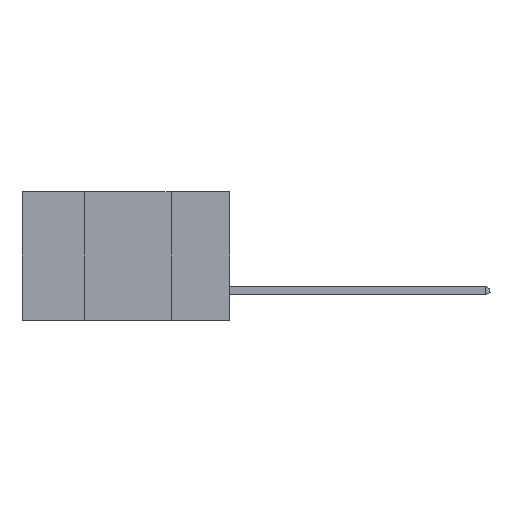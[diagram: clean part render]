
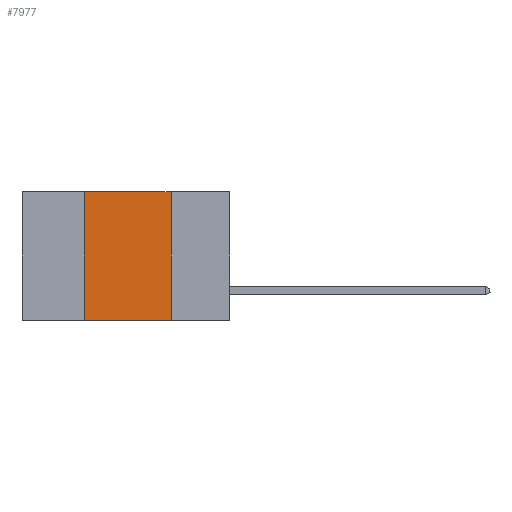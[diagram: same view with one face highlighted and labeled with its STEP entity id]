
A CAD part, left-side view. The second image highlights one B-rep face of the part: STEP entity #7977.
In plain terms, the highlighted planar face has unit normal (-1, 0, 0).
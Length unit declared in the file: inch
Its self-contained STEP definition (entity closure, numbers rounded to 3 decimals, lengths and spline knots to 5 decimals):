
#239 = VERTEX_POINT ( 'NONE', #2856 ) ;
#343 = EDGE_CURVE ( 'NONE', #239, #14109, #8706, .T. ) ;
#652 = VERTEX_POINT ( 'NONE', #15212 ) ;
#1117 = LINE ( 'NONE', #10203, #15800 ) ;
#1654 = VECTOR ( 'NONE', #10891, 39.37008 ) ;
#2674 = DIRECTION ( 'NONE',  ( 0., 0., -1. ) ) ;
#2856 = CARTESIAN_POINT ( 'NONE',  ( 0., 0.42, 0. ) ) ;
#3702 = ORIENTED_EDGE ( 'NONE', *, *, #10461, .T. ) ;
#3915 = ORIENTED_EDGE ( 'NONE', *, *, #6969, .F. ) ;
#4906 = AXIS2_PLACEMENT_3D ( 'NONE', #9082, #7619, #2674 ) ;
#5778 = CARTESIAN_POINT ( 'NONE',  ( 0., 0.17, 0. ) ) ;
#5860 = CARTESIAN_POINT ( 'NONE',  ( 0., 0.6, -0.37 ) ) ;
#6131 = FACE_OUTER_BOUND ( 'NONE', #7118, .T. ) ;
#6328 = PLANE ( 'NONE',  #4906 ) ;
#6969 = EDGE_CURVE ( 'NONE', #14109, #652, #8260, .T. ) ;
#7118 = EDGE_LOOP ( 'NONE', ( #3915, #11951, #8737, #3702 ) ) ;
#7619 = DIRECTION ( 'NONE',  ( 1., 0., 0. ) ) ;
#7655 = EDGE_CURVE ( 'NONE', #8499, #239, #1117, .T. ) ;
#7977 = ADVANCED_FACE ( 'NONE', ( #6131 ), #6328, .F. ) ;
#8260 = LINE ( 'NONE', #14717, #9081 ) ;
#8499 = VERTEX_POINT ( 'NONE', #16238 ) ;
#8671 = DIRECTION ( 'NONE',  ( 0., -1., 0. ) ) ;
#8706 = LINE ( 'NONE', #15983, #1654 ) ;
#8737 = ORIENTED_EDGE ( 'NONE', *, *, #7655, .F. ) ;
#9073 = LINE ( 'NONE', #5860, #13459 ) ;
#9081 = VECTOR ( 'NONE', #12280, 39.37008 ) ;
#9082 = CARTESIAN_POINT ( 'NONE',  ( 0., 0.6, 0. ) ) ;
#10203 = CARTESIAN_POINT ( 'NONE',  ( 0., 0.42, 0. ) ) ;
#10461 = EDGE_CURVE ( 'NONE', #8499, #652, #9073, .T. ) ;
#10891 = DIRECTION ( 'NONE',  ( 0., -1., 0. ) ) ;
#11951 = ORIENTED_EDGE ( 'NONE', *, *, #343, .F. ) ;
#12280 = DIRECTION ( 'NONE',  ( 0., 0., -1. ) ) ;
#13459 = VECTOR ( 'NONE', #8671, 39.37008 ) ;
#14109 = VERTEX_POINT ( 'NONE', #5778 ) ;
#14717 = CARTESIAN_POINT ( 'NONE',  ( 0., 0.17, 0. ) ) ;
#15212 = CARTESIAN_POINT ( 'NONE',  ( 0., 0.17, -0.37 ) ) ;
#15800 = VECTOR ( 'NONE', #15895, 39.37008 ) ;
#15895 = DIRECTION ( 'NONE',  ( 0., 0., 1. ) ) ;
#15983 = CARTESIAN_POINT ( 'NONE',  ( 0., 0.6, 0. ) ) ;
#16238 = CARTESIAN_POINT ( 'NONE',  ( 0., 0.42, -0.37 ) ) ;
